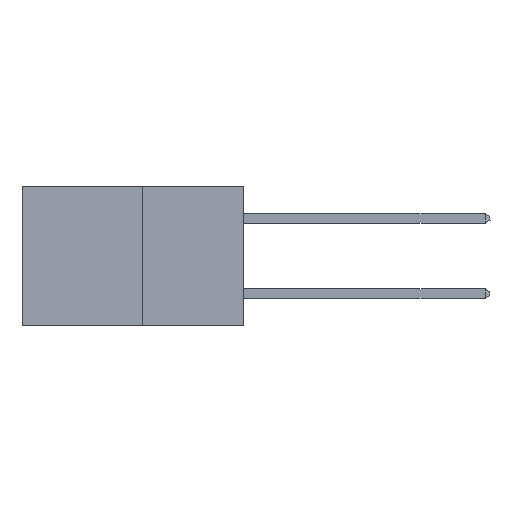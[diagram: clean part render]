
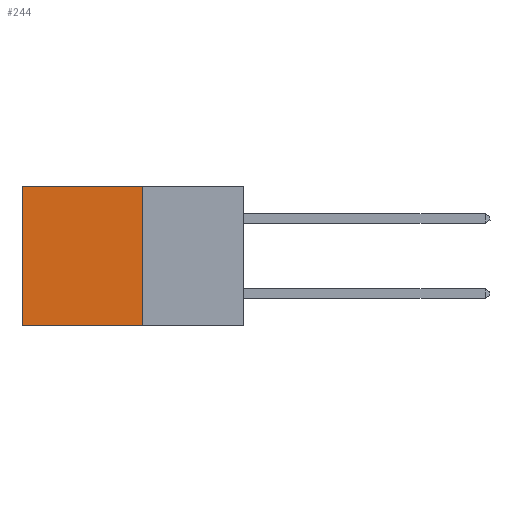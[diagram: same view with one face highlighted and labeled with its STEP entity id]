
A CAD part, left-side view. The second image highlights one B-rep face of the part: STEP entity #244.
In plain terms, the highlighted planar face has unit normal (-1, 0, 0).
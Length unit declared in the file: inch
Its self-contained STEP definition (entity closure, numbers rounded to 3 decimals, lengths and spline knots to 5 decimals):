
#178 = CARTESIAN_POINT ( 'NONE',  ( 0.277, 0.27, -0.37 ) ) ;
#244 = ADVANCED_FACE ( 'NONE', ( #6004 ), #1474, .F. ) ;
#500 = VECTOR ( 'NONE', #6200, 39.37008 ) ;
#796 = LINE ( 'NONE', #1332, #2693 ) ;
#1332 = CARTESIAN_POINT ( 'NONE',  ( 0.277, 0.27, -0.37 ) ) ;
#1366 = ORIENTED_EDGE ( 'NONE', *, *, #4063, .F. ) ;
#1474 = PLANE ( 'NONE',  #5975 ) ;
#1542 = ORIENTED_EDGE ( 'NONE', *, *, #7624, .F. ) ;
#1598 = CARTESIAN_POINT ( 'NONE',  ( 0.277, 0.27, -0.37 ) ) ;
#1995 = VECTOR ( 'NONE', #7238, 39.37008 ) ;
#2239 = CARTESIAN_POINT ( 'NONE',  ( 0.277, 0.27, -0.37 ) ) ;
#2375 = CARTESIAN_POINT ( 'NONE',  ( 0.277, 0.59, -0.37 ) ) ;
#2693 = VECTOR ( 'NONE', #5886, 39.37008 ) ;
#2837 = ORIENTED_EDGE ( 'NONE', *, *, #3792, .T. ) ;
#2883 = VERTEX_POINT ( 'NONE', #1598 ) ;
#3062 = VERTEX_POINT ( 'NONE', #7021 ) ;
#3792 = EDGE_CURVE ( 'NONE', #5167, #3062, #7131, .T. ) ;
#4063 = EDGE_CURVE ( 'NONE', #8124, #2883, #8408, .T. ) ;
#4288 = CARTESIAN_POINT ( 'NONE',  ( 0.277, 0.27, 0. ) ) ;
#4507 = CARTESIAN_POINT ( 'NONE',  ( 0.277, 0.27, 0. ) ) ;
#4768 = ORIENTED_EDGE ( 'NONE', *, *, #6707, .T. ) ;
#5167 = VERTEX_POINT ( 'NONE', #5848 ) ;
#5761 = DIRECTION ( 'NONE',  ( 0., 0., -1. ) ) ;
#5816 = LINE ( 'NONE', #4288, #500 ) ;
#5830 = DIRECTION ( 'NONE',  ( 0., 0., -1. ) ) ;
#5848 = CARTESIAN_POINT ( 'NONE',  ( 0.277, 0.59, 0. ) ) ;
#5886 = DIRECTION ( 'NONE',  ( 0., 1., 0. ) ) ;
#5975 = AXIS2_PLACEMENT_3D ( 'NONE', #2239, #7068, #5761 ) ;
#6004 = FACE_OUTER_BOUND ( 'NONE', #7002, .T. ) ;
#6200 = DIRECTION ( 'NONE',  ( 0., 1., 0. ) ) ;
#6628 = VECTOR ( 'NONE', #5830, 39.37008 ) ;
#6707 = EDGE_CURVE ( 'NONE', #8124, #5167, #5816, .T. ) ;
#7002 = EDGE_LOOP ( 'NONE', ( #2837, #1542, #1366, #4768 ) ) ;
#7021 = CARTESIAN_POINT ( 'NONE',  ( 0.277, 0.59, -0.37 ) ) ;
#7068 = DIRECTION ( 'NONE',  ( 1., 0., 0. ) ) ;
#7131 = LINE ( 'NONE', #2375, #1995 ) ;
#7238 = DIRECTION ( 'NONE',  ( 0., 0., -1. ) ) ;
#7624 = EDGE_CURVE ( 'NONE', #2883, #3062, #796, .T. ) ;
#8124 = VERTEX_POINT ( 'NONE', #4507 ) ;
#8408 = LINE ( 'NONE', #178, #6628 ) ;
